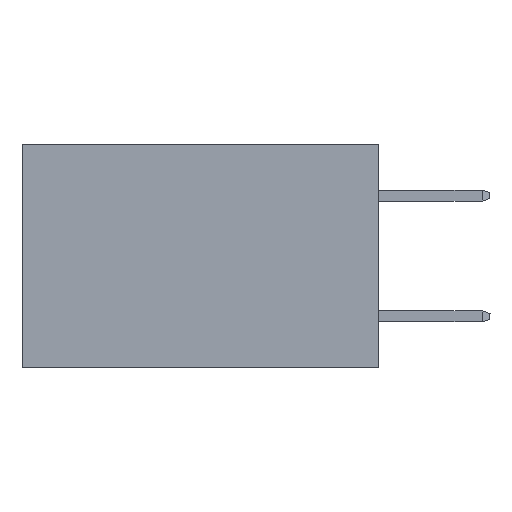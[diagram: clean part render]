
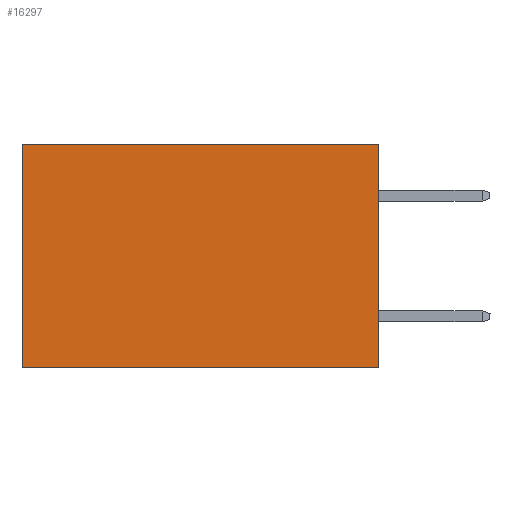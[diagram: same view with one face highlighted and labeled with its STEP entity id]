
A CAD part, left-side view. The second image highlights one B-rep face of the part: STEP entity #16297.
In plain terms, the highlighted planar face has unit normal (-1, 0, 0).
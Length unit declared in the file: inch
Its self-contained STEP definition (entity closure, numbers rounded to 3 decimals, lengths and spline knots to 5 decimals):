
#309 = DIRECTION ( 'NONE',  ( 1., 0., 0. ) ) ;
#433 = VERTEX_POINT ( 'NONE', #7013 ) ;
#574 = CARTESIAN_POINT ( 'NONE',  ( 0.277, 0., 0. ) ) ;
#1560 = VECTOR ( 'NONE', #27035, 39.37008 ) ;
#2789 = CARTESIAN_POINT ( 'NONE',  ( 0.277, 0., -0.37 ) ) ;
#3204 = EDGE_CURVE ( 'NONE', #6451, #16180, #16274, .T. ) ;
#3898 = ORIENTED_EDGE ( 'NONE', *, *, #28234, .F. ) ;
#4100 = VECTOR ( 'NONE', #22926, 39.37008 ) ;
#4353 = VECTOR ( 'NONE', #13741, 39.37008 ) ;
#4697 = ORIENTED_EDGE ( 'NONE', *, *, #3204, .T. ) ;
#6451 = VERTEX_POINT ( 'NONE', #15877 ) ;
#7013 = CARTESIAN_POINT ( 'NONE',  ( 0.277, 0., 0. ) ) ;
#7340 = VERTEX_POINT ( 'NONE', #2789 ) ;
#9205 = FACE_OUTER_BOUND ( 'NONE', #24304, .T. ) ;
#10848 = ORIENTED_EDGE ( 'NONE', *, *, #26516, .F. ) ;
#11773 = LINE ( 'NONE', #574, #23637 ) ;
#11802 = CARTESIAN_POINT ( 'NONE',  ( 0.277, 0., -0.37 ) ) ;
#13671 = PLANE ( 'NONE',  #16277 ) ;
#13741 = DIRECTION ( 'NONE',  ( 0., 0., -1. ) ) ;
#13762 = CARTESIAN_POINT ( 'NONE',  ( 0.277, 0., -0.37 ) ) ;
#15388 = ORIENTED_EDGE ( 'NONE', *, *, #21040, .T. ) ;
#15877 = CARTESIAN_POINT ( 'NONE',  ( 0.277, 0.59, 0. ) ) ;
#15930 = DIRECTION ( 'NONE',  ( 0., 0., -1. ) ) ;
#16180 = VERTEX_POINT ( 'NONE', #22783 ) ;
#16209 = DIRECTION ( 'NONE',  ( 0., 1., 0. ) ) ;
#16274 = LINE ( 'NONE', #16657, #4353 ) ;
#16277 = AXIS2_PLACEMENT_3D ( 'NONE', #20355, #309, #15930 ) ;
#16297 = ADVANCED_FACE ( 'NONE', ( #9205 ), #13671, .F. ) ;
#16657 = CARTESIAN_POINT ( 'NONE',  ( 0.277, 0.59, -0.37 ) ) ;
#20355 = CARTESIAN_POINT ( 'NONE',  ( 0.277, 0., -0.37 ) ) ;
#21040 = EDGE_CURVE ( 'NONE', #433, #6451, #11773, .T. ) ;
#21963 = LINE ( 'NONE', #11802, #4100 ) ;
#22783 = CARTESIAN_POINT ( 'NONE',  ( 0.277, 0.59, -0.37 ) ) ;
#22926 = DIRECTION ( 'NONE',  ( 0., 0., -1. ) ) ;
#23637 = VECTOR ( 'NONE', #16209, 39.37008 ) ;
#24304 = EDGE_LOOP ( 'NONE', ( #4697, #3898, #10848, #15388 ) ) ;
#24580 = LINE ( 'NONE', #13762, #1560 ) ;
#26516 = EDGE_CURVE ( 'NONE', #433, #7340, #21963, .T. ) ;
#27035 = DIRECTION ( 'NONE',  ( 0., 1., 0. ) ) ;
#28234 = EDGE_CURVE ( 'NONE', #7340, #16180, #24580, .T. ) ;
